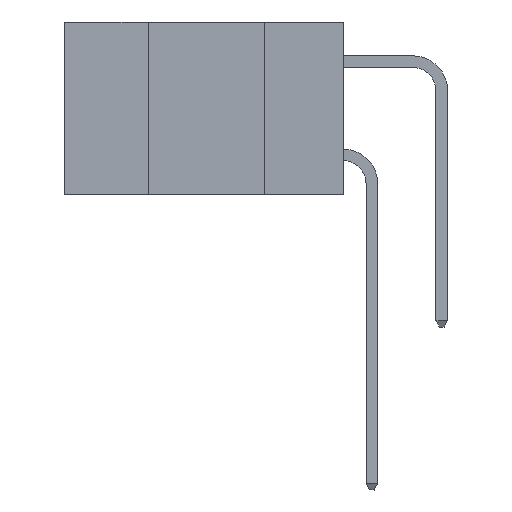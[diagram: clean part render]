
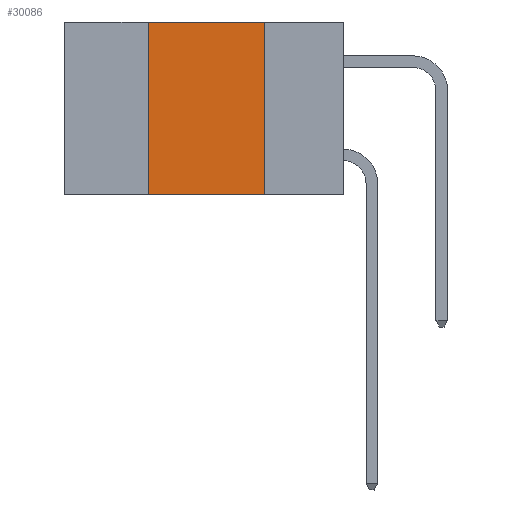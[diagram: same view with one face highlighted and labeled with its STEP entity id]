
A CAD part, left-side view. The second image highlights one B-rep face of the part: STEP entity #30086.
In plain terms, the highlighted planar face has unit normal (-1, 0, 0).
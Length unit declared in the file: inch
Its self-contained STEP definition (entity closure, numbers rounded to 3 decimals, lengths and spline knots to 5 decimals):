
#1332 = ORIENTED_EDGE ( 'NONE', *, *, #26158, .F. ) ;
#2151 = CARTESIAN_POINT ( 'NONE',  ( 0., 0.6, -0.37 ) ) ;
#2759 = CARTESIAN_POINT ( 'NONE',  ( 0., 0.17, -0.37 ) ) ;
#3909 = LINE ( 'NONE', #11547, #32795 ) ;
#4531 = DIRECTION ( 'NONE',  ( 0., -1., 0. ) ) ;
#4691 = CARTESIAN_POINT ( 'NONE',  ( 0., 0.42, 0. ) ) ;
#4993 = DIRECTION ( 'NONE',  ( 0., -1., 0. ) ) ;
#6583 = ORIENTED_EDGE ( 'NONE', *, *, #14448, .F. ) ;
#7311 = VERTEX_POINT ( 'NONE', #23611 ) ;
#7363 = LINE ( 'NONE', #15685, #20485 ) ;
#7527 = DIRECTION ( 'NONE',  ( 0., 0., 1. ) ) ;
#11103 = LINE ( 'NONE', #2151, #24194 ) ;
#11547 = CARTESIAN_POINT ( 'NONE',  ( 0., 0.17, 0. ) ) ;
#13037 = VECTOR ( 'NONE', #7527, 39.37008 ) ;
#13369 = CARTESIAN_POINT ( 'NONE',  ( 0., 0.6, 0. ) ) ;
#13674 = VERTEX_POINT ( 'NONE', #34957 ) ;
#14448 = EDGE_CURVE ( 'NONE', #7311, #13674, #7363, .T. ) ;
#15685 = CARTESIAN_POINT ( 'NONE',  ( 0., 0.6, 0. ) ) ;
#16145 = DIRECTION ( 'NONE',  ( 0., 0., -1. ) ) ;
#18720 = CARTESIAN_POINT ( 'NONE',  ( 0., 0.42, -0.37 ) ) ;
#20281 = VERTEX_POINT ( 'NONE', #18720 ) ;
#20485 = VECTOR ( 'NONE', #4531, 39.37008 ) ;
#20810 = AXIS2_PLACEMENT_3D ( 'NONE', #13369, #32920, #16145 ) ;
#20994 = EDGE_CURVE ( 'NONE', #20281, #31332, #11103, .T. ) ;
#23611 = CARTESIAN_POINT ( 'NONE',  ( 0., 0.42, 0. ) ) ;
#24194 = VECTOR ( 'NONE', #4993, 39.37008 ) ;
#26158 = EDGE_CURVE ( 'NONE', #13674, #31332, #3909, .T. ) ;
#26394 = FACE_OUTER_BOUND ( 'NONE', #28704, .T. ) ;
#27246 = PLANE ( 'NONE',  #20810 ) ;
#28704 = EDGE_LOOP ( 'NONE', ( #1332, #6583, #36312, #30639 ) ) ;
#30086 = ADVANCED_FACE ( 'NONE', ( #26394 ), #27246, .F. ) ;
#30639 = ORIENTED_EDGE ( 'NONE', *, *, #20994, .T. ) ;
#31332 = VERTEX_POINT ( 'NONE', #2759 ) ;
#31794 = EDGE_CURVE ( 'NONE', #20281, #7311, #35333, .T. ) ;
#32795 = VECTOR ( 'NONE', #34065, 39.37008 ) ;
#32920 = DIRECTION ( 'NONE',  ( 1., 0., 0. ) ) ;
#34065 = DIRECTION ( 'NONE',  ( 0., 0., -1. ) ) ;
#34957 = CARTESIAN_POINT ( 'NONE',  ( 0., 0.17, 0. ) ) ;
#35333 = LINE ( 'NONE', #4691, #13037 ) ;
#36312 = ORIENTED_EDGE ( 'NONE', *, *, #31794, .F. ) ;
